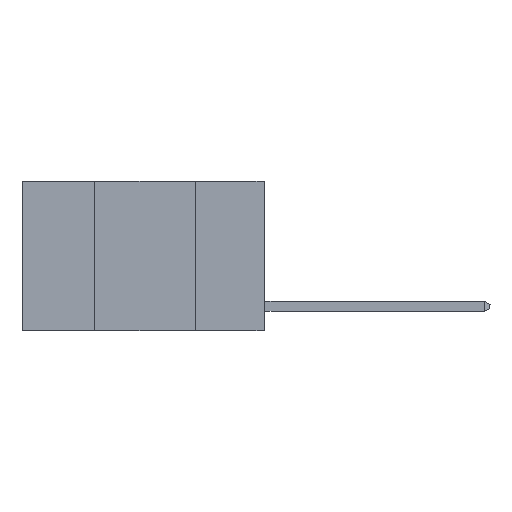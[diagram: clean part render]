
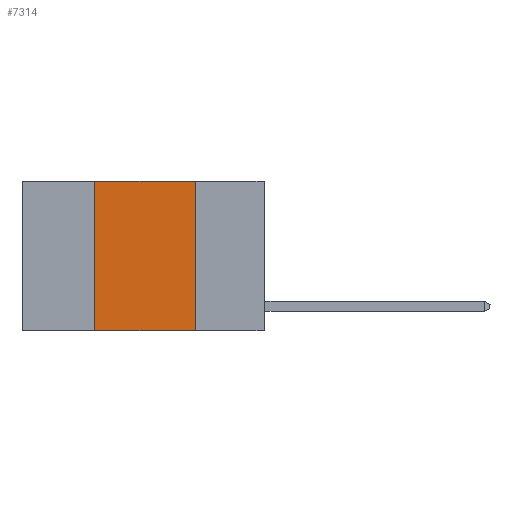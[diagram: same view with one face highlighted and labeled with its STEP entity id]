
A CAD part, left-side view. The second image highlights one B-rep face of the part: STEP entity #7314.
In plain terms, the highlighted planar face has unit normal (-1, 0, 0).
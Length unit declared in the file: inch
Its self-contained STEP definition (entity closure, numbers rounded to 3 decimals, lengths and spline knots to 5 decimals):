
#323 = CARTESIAN_POINT ( 'NONE',  ( 0., 0.6, 0. ) ) ;
#402 = ORIENTED_EDGE ( 'NONE', *, *, #1724, .T. ) ;
#1269 = LINE ( 'NONE', #13632, #2890 ) ;
#1297 = VERTEX_POINT ( 'NONE', #2492 ) ;
#1724 = EDGE_CURVE ( 'NONE', #1297, #14382, #1269, .T. ) ;
#2266 = DIRECTION ( 'NONE',  ( 1., 0., 0. ) ) ;
#2312 = FACE_OUTER_BOUND ( 'NONE', #11494, .T. ) ;
#2376 = CARTESIAN_POINT ( 'NONE',  ( 0., 0.6, 0. ) ) ;
#2492 = CARTESIAN_POINT ( 'NONE',  ( 0., 0.42, -0.37 ) ) ;
#2890 = VECTOR ( 'NONE', #14738, 39.37008 ) ;
#2926 = CARTESIAN_POINT ( 'NONE',  ( 0., 0.17, 0. ) ) ;
#3362 = VERTEX_POINT ( 'NONE', #2926 ) ;
#3724 = CARTESIAN_POINT ( 'NONE',  ( 0., 0.17, 0. ) ) ;
#4859 = DIRECTION ( 'NONE',  ( 0., -1., 0. ) ) ;
#5647 = PLANE ( 'NONE',  #13455 ) ;
#6431 = ORIENTED_EDGE ( 'NONE', *, *, #6877, .F. ) ;
#6504 = VECTOR ( 'NONE', #11742, 39.37008 ) ;
#6877 = EDGE_CURVE ( 'NONE', #1297, #13628, #11641, .T. ) ;
#7154 = ORIENTED_EDGE ( 'NONE', *, *, #11150, .F. ) ;
#7314 = ADVANCED_FACE ( 'NONE', ( #2312 ), #5647, .F. ) ;
#8140 = CARTESIAN_POINT ( 'NONE',  ( 0., 0.42, 0. ) ) ;
#8766 = VECTOR ( 'NONE', #4859, 39.37008 ) ;
#9205 = LINE ( 'NONE', #3724, #6504 ) ;
#9405 = DIRECTION ( 'NONE',  ( 0., 0., 1. ) ) ;
#9922 = ORIENTED_EDGE ( 'NONE', *, *, #12774, .F. ) ;
#10178 = VECTOR ( 'NONE', #9405, 39.37008 ) ;
#11150 = EDGE_CURVE ( 'NONE', #3362, #14382, #9205, .T. ) ;
#11494 = EDGE_LOOP ( 'NONE', ( #7154, #9922, #6431, #402 ) ) ;
#11641 = LINE ( 'NONE', #8140, #10178 ) ;
#11742 = DIRECTION ( 'NONE',  ( 0., 0., -1. ) ) ;
#12189 = LINE ( 'NONE', #323, #8766 ) ;
#12721 = DIRECTION ( 'NONE',  ( 0., 0., -1. ) ) ;
#12774 = EDGE_CURVE ( 'NONE', #13628, #3362, #12189, .T. ) ;
#12902 = CARTESIAN_POINT ( 'NONE',  ( 0., 0.17, -0.37 ) ) ;
#13415 = CARTESIAN_POINT ( 'NONE',  ( 0., 0.42, 0. ) ) ;
#13455 = AXIS2_PLACEMENT_3D ( 'NONE', #2376, #2266, #12721 ) ;
#13628 = VERTEX_POINT ( 'NONE', #13415 ) ;
#13632 = CARTESIAN_POINT ( 'NONE',  ( 0., 0.6, -0.37 ) ) ;
#14382 = VERTEX_POINT ( 'NONE', #12902 ) ;
#14738 = DIRECTION ( 'NONE',  ( 0., -1., 0. ) ) ;
